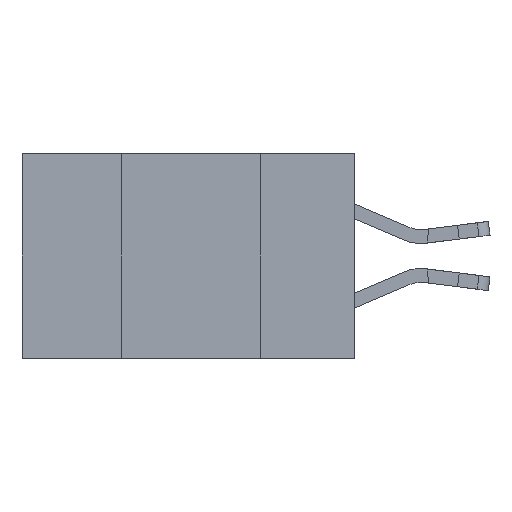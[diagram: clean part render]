
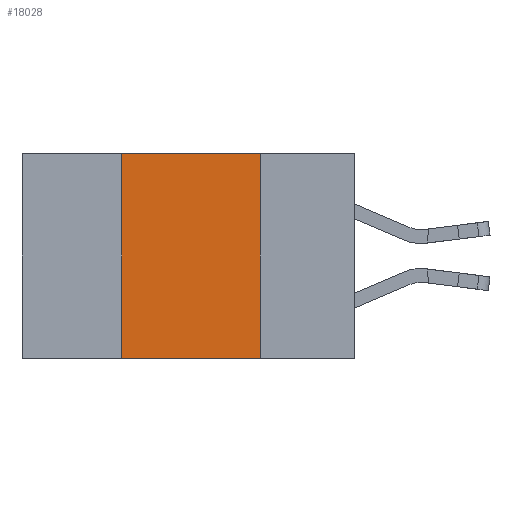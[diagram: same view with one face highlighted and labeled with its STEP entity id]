
A CAD part, left-side view. The second image highlights one B-rep face of the part: STEP entity #18028.
In plain terms, the highlighted planar face has unit normal (-1, 0, 0).
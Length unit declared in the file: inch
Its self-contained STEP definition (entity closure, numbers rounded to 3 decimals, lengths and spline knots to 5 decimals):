
#179 = EDGE_CURVE ( 'NONE', #1298, #20743, #9556, .T. ) ;
#845 = ORIENTED_EDGE ( 'NONE', *, *, #179, .T. ) ;
#962 = LINE ( 'NONE', #6448, #10705 ) ;
#1298 = VERTEX_POINT ( 'NONE', #1386 ) ;
#1386 = CARTESIAN_POINT ( 'NONE',  ( 0., 0.42, -0.37 ) ) ;
#2405 = CARTESIAN_POINT ( 'NONE',  ( 0., 0.6, 0. ) ) ;
#2647 = DIRECTION ( 'NONE',  ( 0., 0., 1. ) ) ;
#5067 = ORIENTED_EDGE ( 'NONE', *, *, #7665, .F. ) ;
#6210 = VECTOR ( 'NONE', #10626, 39.37008 ) ;
#6448 = CARTESIAN_POINT ( 'NONE',  ( 0., 0.17, 0. ) ) ;
#7383 = CARTESIAN_POINT ( 'NONE',  ( 0., 0.6, 0. ) ) ;
#7665 = EDGE_CURVE ( 'NONE', #13852, #17119, #17663, .T. ) ;
#8517 = CARTESIAN_POINT ( 'NONE',  ( 0., 0.42, 0. ) ) ;
#9556 = LINE ( 'NONE', #17769, #19063 ) ;
#9740 = AXIS2_PLACEMENT_3D ( 'NONE', #7383, #11625, #25876 ) ;
#10626 = DIRECTION ( 'NONE',  ( 0., -1., 0. ) ) ;
#10705 = VECTOR ( 'NONE', #22803, 39.37008 ) ;
#11625 = DIRECTION ( 'NONE',  ( 1., 0., 0. ) ) ;
#13852 = VERTEX_POINT ( 'NONE', #8517 ) ;
#15775 = VECTOR ( 'NONE', #2647, 39.37008 ) ;
#15922 = ORIENTED_EDGE ( 'NONE', *, *, #20468, .F. ) ;
#16402 = LINE ( 'NONE', #18988, #15775 ) ;
#16666 = EDGE_LOOP ( 'NONE', ( #26190, #5067, #15922, #845 ) ) ;
#16848 = CARTESIAN_POINT ( 'NONE',  ( 0., 0.17, 0. ) ) ;
#17119 = VERTEX_POINT ( 'NONE', #16848 ) ;
#17663 = LINE ( 'NONE', #2405, #6210 ) ;
#17769 = CARTESIAN_POINT ( 'NONE',  ( 0., 0.6, -0.37 ) ) ;
#18028 = ADVANCED_FACE ( 'NONE', ( #20591 ), #19664, .F. ) ;
#18988 = CARTESIAN_POINT ( 'NONE',  ( 0., 0.42, 0. ) ) ;
#19063 = VECTOR ( 'NONE', #19710, 39.37008 ) ;
#19077 = EDGE_CURVE ( 'NONE', #17119, #20743, #962, .T. ) ;
#19664 = PLANE ( 'NONE',  #9740 ) ;
#19710 = DIRECTION ( 'NONE',  ( 0., -1., 0. ) ) ;
#20468 = EDGE_CURVE ( 'NONE', #1298, #13852, #16402, .T. ) ;
#20591 = FACE_OUTER_BOUND ( 'NONE', #16666, .T. ) ;
#20743 = VERTEX_POINT ( 'NONE', #23931 ) ;
#22803 = DIRECTION ( 'NONE',  ( 0., 0., -1. ) ) ;
#23931 = CARTESIAN_POINT ( 'NONE',  ( 0., 0.17, -0.37 ) ) ;
#25876 = DIRECTION ( 'NONE',  ( 0., 0., -1. ) ) ;
#26190 = ORIENTED_EDGE ( 'NONE', *, *, #19077, .F. ) ;
